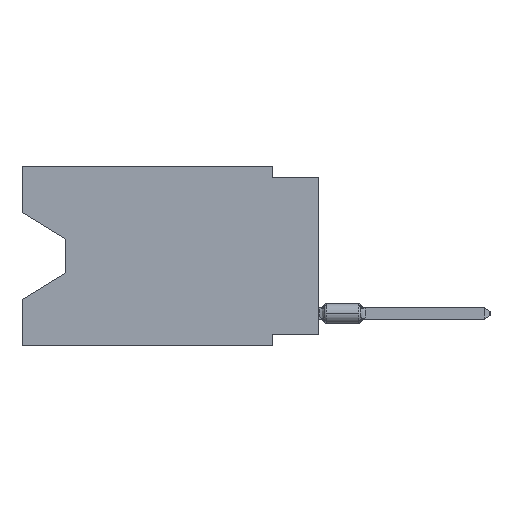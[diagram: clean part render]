
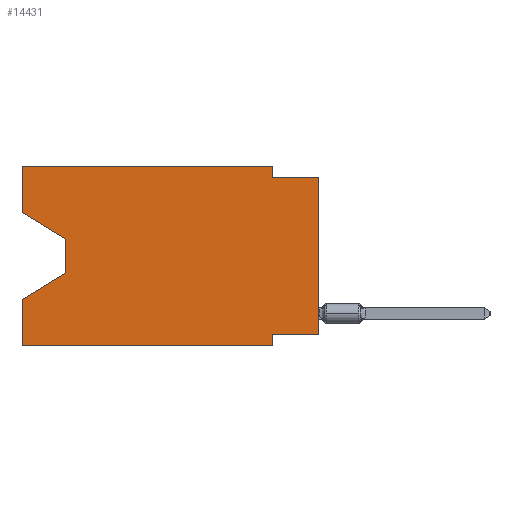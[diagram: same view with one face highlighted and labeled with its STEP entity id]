
A CAD part, left-side view. The second image highlights one B-rep face of the part: STEP entity #14431.
In plain terms, the highlighted planar face has unit normal (-1, 0, 0).
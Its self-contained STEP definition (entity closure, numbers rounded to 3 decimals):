
#37 = DIRECTION ( 'NONE',  ( 0., 0., 1. ) ) ;
#177 = VECTOR ( 'NONE', #37, 1000. ) ;
#535 = ORIENTED_EDGE ( 'NONE', *, *, #24800, .F. ) ;
#1099 = CARTESIAN_POINT ( 'NONE',  ( 0., 16.383, 0. ) ) ;
#1267 = VECTOR ( 'NONE', #32487, 1000. ) ;
#1721 = LINE ( 'NONE', #7018, #18506 ) ;
#1943 = CARTESIAN_POINT ( 'NONE',  ( 0., 2.54, -9.906 ) ) ;
#2292 = DIRECTION ( 'NONE',  ( 0., 0., -1. ) ) ;
#2414 = CARTESIAN_POINT ( 'NONE',  ( 0., 16.383, -7.36 ) ) ;
#3882 = LINE ( 'NONE', #36323, #24012 ) ;
#4048 = DIRECTION ( 'NONE',  ( 0., -1., 0. ) ) ;
#4481 = EDGE_CURVE ( 'NONE', #15956, #46431, #4813, .T. ) ;
#4700 = EDGE_LOOP ( 'NONE', ( #46769, #25330, #26955, #36618, #50394, #26423, #51464, #31106, #535, #7863, #49653, #51620 ) ) ;
#4813 = LINE ( 'NONE', #44415, #177 ) ;
#5835 = LINE ( 'NONE', #30561, #18356 ) ;
#6101 = EDGE_CURVE ( 'NONE', #10912, #41365, #6183, .T. ) ;
#6183 = LINE ( 'NONE', #38610, #1267 ) ;
#6741 = CARTESIAN_POINT ( 'NONE',  ( 0., 2.54, 0. ) ) ;
#6886 = EDGE_CURVE ( 'NONE', #47156, #49131, #13774, .T. ) ;
#7018 = CARTESIAN_POINT ( 'NONE',  ( 0., 0., -0.635 ) ) ;
#7863 = ORIENTED_EDGE ( 'NONE', *, *, #11747, .F. ) ;
#8831 = VERTEX_POINT ( 'NONE', #1943 ) ;
#9785 = CARTESIAN_POINT ( 'NONE',  ( 0., 0., -9.271 ) ) ;
#10561 = DIRECTION ( 'NONE',  ( 0., 1., 0. ) ) ;
#10912 = VERTEX_POINT ( 'NONE', #32926 ) ;
#10966 = EDGE_CURVE ( 'NONE', #15956, #43073, #37697, .T. ) ;
#11747 = EDGE_CURVE ( 'NONE', #38552, #16105, #41492, .T. ) ;
#12138 = VECTOR ( 'NONE', #4048, 1000. ) ;
#12265 = CARTESIAN_POINT ( 'NONE',  ( 0., 13.97, -5.893 ) ) ;
#13305 = DIRECTION ( 'NONE',  ( 0., 0., -1. ) ) ;
#13774 = LINE ( 'NONE', #9785, #26770 ) ;
#14431 = ADVANCED_FACE ( 'NONE', ( #37936 ), #46395, .F. ) ;
#14691 = DIRECTION ( 'NONE',  ( 0., 0., 1. ) ) ;
#15388 = VERTEX_POINT ( 'NONE', #28147 ) ;
#15956 = VERTEX_POINT ( 'NONE', #38197 ) ;
#16105 = VERTEX_POINT ( 'NONE', #18795 ) ;
#16980 = EDGE_CURVE ( 'NONE', #15388, #41365, #27693, .T. ) ;
#18356 = VECTOR ( 'NONE', #41739, 1000. ) ;
#18465 = VECTOR ( 'NONE', #14691, 1000. ) ;
#18506 = VECTOR ( 'NONE', #34681, 1000. ) ;
#18795 = CARTESIAN_POINT ( 'NONE',  ( 0., 2.54, -0.635 ) ) ;
#22916 = VECTOR ( 'NONE', #44853, 1000. ) ;
#24012 = VECTOR ( 'NONE', #28352, 1000. ) ;
#24800 = EDGE_CURVE ( 'NONE', #16105, #26545, #1721, .T. ) ;
#25295 = CARTESIAN_POINT ( 'NONE',  ( 0., 2.54, 0. ) ) ;
#25330 = ORIENTED_EDGE ( 'NONE', *, *, #26606, .T. ) ;
#25976 = CARTESIAN_POINT ( 'NONE',  ( 0., 16.383, 0. ) ) ;
#26423 = ORIENTED_EDGE ( 'NONE', *, *, #46874, .F. ) ;
#26545 = VERTEX_POINT ( 'NONE', #35945 ) ;
#26606 = EDGE_CURVE ( 'NONE', #43073, #15388, #29010, .T. ) ;
#26770 = VECTOR ( 'NONE', #10561, 1000. ) ;
#26955 = ORIENTED_EDGE ( 'NONE', *, *, #16980, .T. ) ;
#27693 = LINE ( 'NONE', #12265, #47994 ) ;
#28147 = CARTESIAN_POINT ( 'NONE',  ( 0., 13.97, -5.893 ) ) ;
#28352 = DIRECTION ( 'NONE',  ( 0., 0., -1. ) ) ;
#28935 = CARTESIAN_POINT ( 'NONE',  ( 0., 16.383, -2.546 ) ) ;
#28992 = EDGE_CURVE ( 'NONE', #46431, #38552, #5835, .T. ) ;
#29010 = LINE ( 'NONE', #48891, #50119 ) ;
#29849 = EDGE_CURVE ( 'NONE', #47156, #26545, #34899, .T. ) ;
#30561 = CARTESIAN_POINT ( 'NONE',  ( 0., 16.383, 0. ) ) ;
#31106 = ORIENTED_EDGE ( 'NONE', *, *, #29849, .T. ) ;
#32487 = DIRECTION ( 'NONE',  ( 0., 0., 1. ) ) ;
#32926 = CARTESIAN_POINT ( 'NONE',  ( 0., 16.383, -9.906 ) ) ;
#33277 = DIRECTION ( 'NONE',  ( 0., 0., -1. ) ) ;
#34098 = EDGE_CURVE ( 'NONE', #10912, #8831, #40457, .T. ) ;
#34681 = DIRECTION ( 'NONE',  ( 0., -1., 0. ) ) ;
#34899 = LINE ( 'NONE', #51058, #18465 ) ;
#35945 = CARTESIAN_POINT ( 'NONE',  ( 0., 0., -0.635 ) ) ;
#36323 = CARTESIAN_POINT ( 'NONE',  ( 0., 2.54, -9.906 ) ) ;
#36618 = ORIENTED_EDGE ( 'NONE', *, *, #6101, .F. ) ;
#36717 = DIRECTION ( 'NONE',  ( 0., 0.855, -0.519 ) ) ;
#36875 = AXIS2_PLACEMENT_3D ( 'NONE', #25976, #38960, #2292 ) ;
#37697 = LINE ( 'NONE', #28935, #22916 ) ;
#37936 = FACE_OUTER_BOUND ( 'NONE', #4700, .T. ) ;
#38197 = CARTESIAN_POINT ( 'NONE',  ( 0., 16.383, -2.546 ) ) ;
#38552 = VERTEX_POINT ( 'NONE', #6741 ) ;
#38610 = CARTESIAN_POINT ( 'NONE',  ( 0., 16.383, 0. ) ) ;
#38730 = CARTESIAN_POINT ( 'NONE',  ( 0., 13.97, -4.013 ) ) ;
#38960 = DIRECTION ( 'NONE',  ( 1., 0., 0. ) ) ;
#40457 = LINE ( 'NONE', #52384, #12138 ) ;
#41365 = VERTEX_POINT ( 'NONE', #2414 ) ;
#41492 = LINE ( 'NONE', #25295, #49034 ) ;
#41739 = DIRECTION ( 'NONE',  ( 0., -1., 0. ) ) ;
#42263 = CARTESIAN_POINT ( 'NONE',  ( 0., 2.54, -9.271 ) ) ;
#43073 = VERTEX_POINT ( 'NONE', #38730 ) ;
#44415 = CARTESIAN_POINT ( 'NONE',  ( 0., 16.383, 0. ) ) ;
#44853 = DIRECTION ( 'NONE',  ( 0., -0.855, -0.519 ) ) ;
#46395 = PLANE ( 'NONE',  #36875 ) ;
#46431 = VERTEX_POINT ( 'NONE', #1099 ) ;
#46769 = ORIENTED_EDGE ( 'NONE', *, *, #10966, .T. ) ;
#46874 = EDGE_CURVE ( 'NONE', #49131, #8831, #3882, .T. ) ;
#47156 = VERTEX_POINT ( 'NONE', #52424 ) ;
#47994 = VECTOR ( 'NONE', #36717, 1000. ) ;
#48891 = CARTESIAN_POINT ( 'NONE',  ( 0., 13.97, -4.013 ) ) ;
#49034 = VECTOR ( 'NONE', #33277, 1000. ) ;
#49131 = VERTEX_POINT ( 'NONE', #42263 ) ;
#49653 = ORIENTED_EDGE ( 'NONE', *, *, #28992, .F. ) ;
#50119 = VECTOR ( 'NONE', #13305, 1000. ) ;
#50394 = ORIENTED_EDGE ( 'NONE', *, *, #34098, .T. ) ;
#51058 = CARTESIAN_POINT ( 'NONE',  ( 0., 0., 0. ) ) ;
#51464 = ORIENTED_EDGE ( 'NONE', *, *, #6886, .F. ) ;
#51620 = ORIENTED_EDGE ( 'NONE', *, *, #4481, .F. ) ;
#52384 = CARTESIAN_POINT ( 'NONE',  ( 0., 16.383, -9.906 ) ) ;
#52424 = CARTESIAN_POINT ( 'NONE',  ( 0., 0., -9.271 ) ) ;
